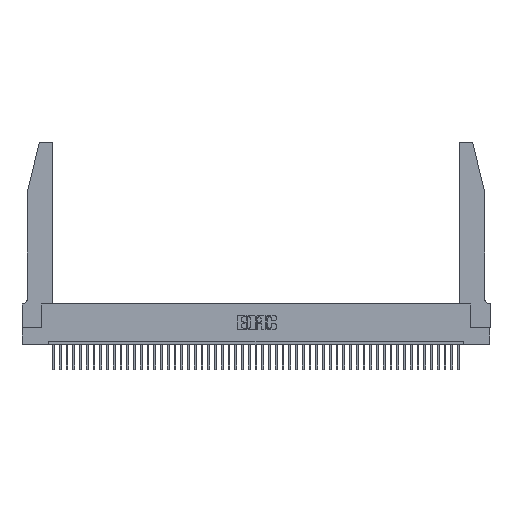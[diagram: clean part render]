
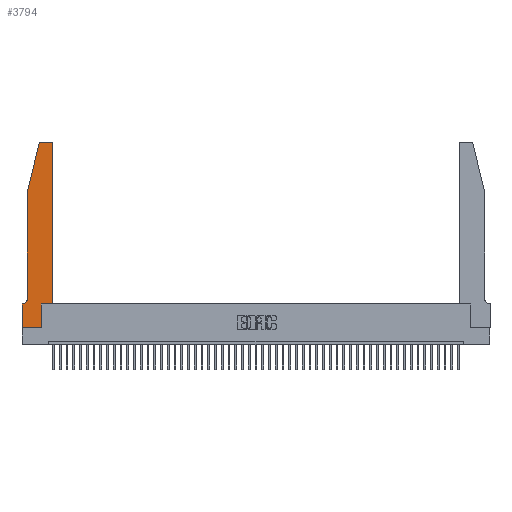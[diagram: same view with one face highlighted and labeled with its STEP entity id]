
A CAD part, top view. The second image highlights one B-rep face of the part: STEP entity #3794.
In plain terms, the highlighted planar face has unit normal (0, 0, 1).
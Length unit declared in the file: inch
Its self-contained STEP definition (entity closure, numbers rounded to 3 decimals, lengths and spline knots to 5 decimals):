
#29 = LINE ( 'NONE', #35956, #10560 ) ;
#106 = LINE ( 'NONE', #35051, #1259 ) ;
#904 = DIRECTION ( 'NONE',  ( 1., 0., 0. ) ) ;
#945 = CIRCLE ( 'NONE', #1455, 0.03 ) ;
#1259 = VECTOR ( 'NONE', #17045, 39.37008 ) ;
#1455 = AXIS2_PLACEMENT_3D ( 'NONE', #2111, #31568, #35306 ) ;
#1480 = VECTOR ( 'NONE', #11376, 39.37008 ) ;
#2111 = CARTESIAN_POINT ( 'NONE',  ( 0.284, 2.72, 0.37 ) ) ;
#2982 = CARTESIAN_POINT ( 'NONE',  ( 0.2865, 0., 0.37 ) ) ;
#3794 = ADVANCED_FACE ( 'NONE', ( #41766 ), #36619, .T. ) ;
#3999 = DIRECTION ( 'NONE',  ( 0., 0., 1. ) ) ;
#5853 = DIRECTION ( 'NONE',  ( 1., 0., 0. ) ) ;
#6369 = ORIENTED_EDGE ( 'NONE', *, *, #36020, .T. ) ;
#6852 = EDGE_CURVE ( 'NONE', #31334, #9885, #23028, .T. ) ;
#7858 = CARTESIAN_POINT ( 'NONE',  ( 0.0055, 0.35, 0.37 ) ) ;
#7865 = VECTOR ( 'NONE', #39968, 39.37008 ) ;
#8609 = CARTESIAN_POINT ( 'NONE',  ( 0.2865, 0.35, 0.37 ) ) ;
#8770 = DIRECTION ( 'NONE',  ( 0., 1., 0. ) ) ;
#9022 = LINE ( 'NONE', #20876, #7865 ) ;
#9885 = VERTEX_POINT ( 'NONE', #41950 ) ;
#10267 = EDGE_CURVE ( 'NONE', #38074, #31361, #26468, .T. ) ;
#10560 = VECTOR ( 'NONE', #5853, 39.37008 ) ;
#10953 = CARTESIAN_POINT ( 'NONE',  ( 0.25487, 2.72718, 0.37 ) ) ;
#10985 = LINE ( 'NONE', #8609, #44586 ) ;
#10999 = DIRECTION ( 'NONE',  ( 0., 0., -1. ) ) ;
#11376 = DIRECTION ( 'NONE',  ( -0.239, -0.971, 0. ) ) ;
#11404 = DIRECTION ( 'NONE',  ( 1., 0., 0. ) ) ;
#11443 = CARTESIAN_POINT ( 'NONE',  ( 0.4505, 0.35, 0.37 ) ) ;
#11466 = CARTESIAN_POINT ( 'NONE',  ( 0.2865, 0.35, 0.37 ) ) ;
#11781 = AXIS2_PLACEMENT_3D ( 'NONE', #12019, #3999, #904 ) ;
#12019 = CARTESIAN_POINT ( 'NONE',  ( 0., 0.35, 0.37 ) ) ;
#12271 = EDGE_CURVE ( 'NONE', #29354, #16492, #29, .T. ) ;
#14918 = ORIENTED_EDGE ( 'NONE', *, *, #38282, .T. ) ;
#15082 = CARTESIAN_POINT ( 'NONE',  ( 0., 0., 0.37 ) ) ;
#16492 = VERTEX_POINT ( 'NONE', #11443 ) ;
#16879 = CARTESIAN_POINT ( 'NONE',  ( 0., 0.35, 0.37 ) ) ;
#16980 = VECTOR ( 'NONE', #26792, 39.37008 ) ;
#17045 = DIRECTION ( 'NONE',  ( 0., -1., 0. ) ) ;
#17562 = ORIENTED_EDGE ( 'NONE', *, *, #33652, .T. ) ;
#18274 = AXIS2_PLACEMENT_3D ( 'NONE', #26362, #33668, #11404 ) ;
#18366 = CARTESIAN_POINT ( 'NONE',  ( 0.0755, 0.35, 0.37 ) ) ;
#20072 = VECTOR ( 'NONE', #43866, 39.37008 ) ;
#20437 = CARTESIAN_POINT ( 'NONE',  ( 0.4205, 2.75, 0.37 ) ) ;
#20739 = CIRCLE ( 'NONE', #25151, 0.07 ) ;
#20876 = CARTESIAN_POINT ( 'NONE',  ( 0.4505, 0.35, 0.37 ) ) ;
#22098 = DIRECTION ( 'NONE',  ( -1., 0., 0. ) ) ;
#23028 = LINE ( 'NONE', #15082, #47943 ) ;
#23227 = CARTESIAN_POINT ( 'NONE',  ( 0.2605, 2.75, 0.37 ) ) ;
#23485 = EDGE_CURVE ( 'NONE', #25334, #26895, #945, .T. ) ;
#24815 = CARTESIAN_POINT ( 'NONE',  ( 0.4505, 2.72, 0.37 ) ) ;
#24983 = ORIENTED_EDGE ( 'NONE', *, *, #10267, .T. ) ;
#25151 = AXIS2_PLACEMENT_3D ( 'NONE', #44220, #10999, #47622 ) ;
#25291 = EDGE_CURVE ( 'NONE', #9885, #31423, #33996, .T. ) ;
#25334 = VERTEX_POINT ( 'NONE', #45310 ) ;
#26362 = CARTESIAN_POINT ( 'NONE',  ( 0.4205, 2.72, 0.37 ) ) ;
#26468 = CIRCLE ( 'NONE', #18274, 0.03 ) ;
#26792 = DIRECTION ( 'NONE',  ( -1., 0., 0. ) ) ;
#26895 = VERTEX_POINT ( 'NONE', #10953 ) ;
#29354 = VERTEX_POINT ( 'NONE', #11466 ) ;
#30516 = ORIENTED_EDGE ( 'NONE', *, *, #23485, .T. ) ;
#30907 = EDGE_CURVE ( 'NONE', #45348, #37001, #20739, .T. ) ;
#31334 = VERTEX_POINT ( 'NONE', #16879 ) ;
#31361 = VERTEX_POINT ( 'NONE', #20437 ) ;
#31423 = VERTEX_POINT ( 'NONE', #2982 ) ;
#31509 = LINE ( 'NONE', #23227, #16980 ) ;
#31568 = DIRECTION ( 'NONE',  ( 0., 0., 1. ) ) ;
#32544 = EDGE_CURVE ( 'NONE', #16492, #38074, #9022, .T. ) ;
#33433 = CARTESIAN_POINT ( 'NONE',  ( 0.0755, 0.42, 0.37 ) ) ;
#33652 = EDGE_CURVE ( 'NONE', #37405, #45348, #106, .T. ) ;
#33668 = DIRECTION ( 'NONE',  ( 0., 0., 1. ) ) ;
#33996 = LINE ( 'NONE', #47088, #20072 ) ;
#34227 = ORIENTED_EDGE ( 'NONE', *, *, #6852, .T. ) ;
#34262 = EDGE_CURVE ( 'NONE', #31361, #25334, #31509, .T. ) ;
#34317 = ORIENTED_EDGE ( 'NONE', *, *, #25291, .T. ) ;
#34407 = LINE ( 'NONE', #18366, #35584 ) ;
#35051 = CARTESIAN_POINT ( 'NONE',  ( 0.0755, 2., 0.37 ) ) ;
#35070 = EDGE_CURVE ( 'NONE', #31423, #29354, #10985, .T. ) ;
#35306 = DIRECTION ( 'NONE',  ( 1., 0., 0. ) ) ;
#35584 = VECTOR ( 'NONE', #22098, 39.37008 ) ;
#35956 = CARTESIAN_POINT ( 'NONE',  ( 0.4505, 0.35, 0.37 ) ) ;
#36020 = EDGE_CURVE ( 'NONE', #26895, #37405, #42726, .T. ) ;
#36619 = PLANE ( 'NONE',  #11781 ) ;
#37001 = VERTEX_POINT ( 'NONE', #7858 ) ;
#37405 = VERTEX_POINT ( 'NONE', #41971 ) ;
#37420 = DIRECTION ( 'NONE',  ( 0., -1., 0. ) ) ;
#37549 = ORIENTED_EDGE ( 'NONE', *, *, #32544, .T. ) ;
#38074 = VERTEX_POINT ( 'NONE', #24815 ) ;
#38282 = EDGE_CURVE ( 'NONE', #37001, #31334, #34407, .T. ) ;
#39968 = DIRECTION ( 'NONE',  ( 0., 1., 0. ) ) ;
#41049 = EDGE_LOOP ( 'NONE', ( #46460, #30516, #6369, #17562, #45874, #14918, #34227, #34317, #47608, #48017, #37549, #24983 ) ) ;
#41766 = FACE_OUTER_BOUND ( 'NONE', #41049, .T. ) ;
#41950 = CARTESIAN_POINT ( 'NONE',  ( 0., 0., 0.37 ) ) ;
#41971 = CARTESIAN_POINT ( 'NONE',  ( 0.0755, 2., 0.37 ) ) ;
#42726 = LINE ( 'NONE', #47688, #1480 ) ;
#43866 = DIRECTION ( 'NONE',  ( 1., 0., 0. ) ) ;
#44220 = CARTESIAN_POINT ( 'NONE',  ( 0.0055, 0.42, 0.37 ) ) ;
#44586 = VECTOR ( 'NONE', #8770, 39.37008 ) ;
#45310 = CARTESIAN_POINT ( 'NONE',  ( 0.284, 2.75, 0.37 ) ) ;
#45348 = VERTEX_POINT ( 'NONE', #33433 ) ;
#45874 = ORIENTED_EDGE ( 'NONE', *, *, #30907, .T. ) ;
#46460 = ORIENTED_EDGE ( 'NONE', *, *, #34262, .T. ) ;
#47088 = CARTESIAN_POINT ( 'NONE',  ( 0., 0., 0.37 ) ) ;
#47608 = ORIENTED_EDGE ( 'NONE', *, *, #35070, .T. ) ;
#47622 = DIRECTION ( 'NONE',  ( -1., 0., 0. ) ) ;
#47688 = CARTESIAN_POINT ( 'NONE',  ( 0.0755, 2., 0.37 ) ) ;
#47943 = VECTOR ( 'NONE', #37420, 39.37008 ) ;
#48017 = ORIENTED_EDGE ( 'NONE', *, *, #12271, .T. ) ;
